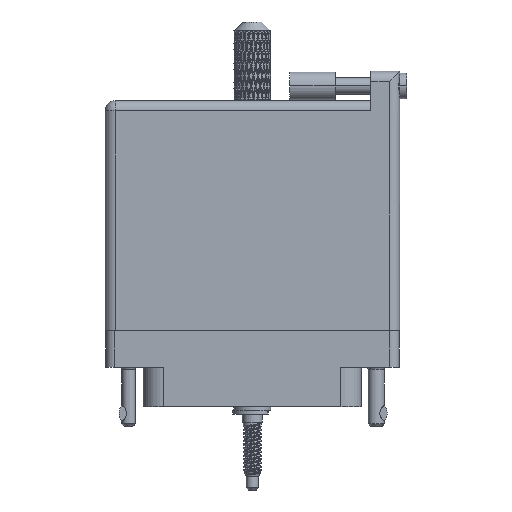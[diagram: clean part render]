
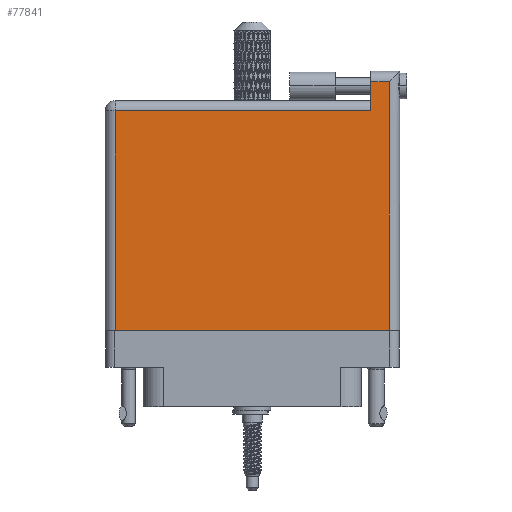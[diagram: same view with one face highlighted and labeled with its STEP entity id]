
A CAD part, front view. The second image highlights one B-rep face of the part: STEP entity #77841.
In plain terms, the highlighted face is planar.
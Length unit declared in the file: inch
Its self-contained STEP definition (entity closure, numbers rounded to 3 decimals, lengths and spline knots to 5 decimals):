
#797 = AXIS2_PLACEMENT_3D ( 'NONE', #28950, #56040, #91653 ) ;
#2466 = VERTEX_POINT ( 'NONE', #64165 ) ;
#3136 = ORIENTED_EDGE ( 'NONE', *, *, #99495, .T. ) ;
#6289 = LINE ( 'NONE', #6969, #58977 ) ;
#6969 = CARTESIAN_POINT ( 'NONE',  ( -1.004, 1.596, 0.4495 ) ) ;
#8138 = LINE ( 'NONE', #91094, #111970 ) ;
#11871 = PLANE ( 'NONE',  #797 ) ;
#13408 = VERTEX_POINT ( 'NONE', #24017 ) ;
#19342 = VERTEX_POINT ( 'NONE', #35663 ) ;
#21701 = EDGE_CURVE ( 'NONE', #56853, #80754, #68148, .T. ) ;
#23378 = CARTESIAN_POINT ( 'NONE',  ( -0.934, -0.1, 0.4495 ) ) ;
#24017 = CARTESIAN_POINT ( 'NONE',  ( 0.807, 1.596, 0.4495 ) ) ;
#25613 = ORIENTED_EDGE ( 'NONE', *, *, #74260, .T. ) ;
#26978 = ORIENTED_EDGE ( 'NONE', *, *, #79634, .T. ) ;
#27271 = ORIENTED_EDGE ( 'NONE', *, *, #21701, .T. ) ;
#28950 = CARTESIAN_POINT ( 'NONE',  ( -1.004, 1.466, 0.4495 ) ) ;
#33632 = LINE ( 'NONE', #95718, #86313 ) ;
#34148 = DIRECTION ( 'NONE',  ( 0., 1., 0. ) ) ;
#35663 = CARTESIAN_POINT ( 'NONE',  ( 0.807, 1.396, 0.4495 ) ) ;
#43052 = VERTEX_POINT ( 'NONE', #74578 ) ;
#43727 = CARTESIAN_POINT ( 'NONE',  ( -1.004, 1.396, 0.4495 ) ) ;
#43791 = ORIENTED_EDGE ( 'NONE', *, *, #59577, .T. ) ;
#44895 = DIRECTION ( 'NONE',  ( 0., -1., 0. ) ) ;
#51412 = EDGE_LOOP ( 'NONE', ( #43791, #25613, #26978, #58460, #3136, #27271 ) ) ;
#53450 = CARTESIAN_POINT ( 'NONE',  ( -0.934, -0.1, 0.4495 ) ) ;
#56040 = DIRECTION ( 'NONE',  ( 0., 0., -1. ) ) ;
#56853 = VERTEX_POINT ( 'NONE', #70923 ) ;
#58460 = ORIENTED_EDGE ( 'NONE', *, *, #112462, .T. ) ;
#58977 = VECTOR ( 'NONE', #87895, 39.37008 ) ;
#59248 = CARTESIAN_POINT ( 'NONE',  ( -1.004, -0.1, 0.4495 ) ) ;
#59577 = EDGE_CURVE ( 'NONE', #80754, #2466, #71367, .T. ) ;
#60408 = DIRECTION ( 'NONE',  ( -1., 0., 0. ) ) ;
#64165 = CARTESIAN_POINT ( 'NONE',  ( 0.934, -0.1, 0.4495 ) ) ;
#67650 = FACE_OUTER_BOUND ( 'NONE', #51412, .T. ) ;
#68148 = LINE ( 'NONE', #53450, #84728 ) ;
#70923 = CARTESIAN_POINT ( 'NONE',  ( -0.934, 1.396, 0.4495 ) ) ;
#71240 = VECTOR ( 'NONE', #111097, 39.37008 ) ;
#71367 = LINE ( 'NONE', #59248, #71240 ) ;
#72909 = VECTOR ( 'NONE', #60408, 39.37008 ) ;
#74260 = EDGE_CURVE ( 'NONE', #2466, #43052, #33632, .T. ) ;
#74578 = CARTESIAN_POINT ( 'NONE',  ( 0.934, 1.596, 0.4495 ) ) ;
#77841 = ADVANCED_FACE ( 'NONE', ( #67650 ), #11871, .F. ) ;
#79634 = EDGE_CURVE ( 'NONE', #43052, #13408, #6289, .T. ) ;
#80754 = VERTEX_POINT ( 'NONE', #23378 ) ;
#84728 = VECTOR ( 'NONE', #44895, 39.37008 ) ;
#86313 = VECTOR ( 'NONE', #34148, 39.37008 ) ;
#87895 = DIRECTION ( 'NONE',  ( -1., 0., 0. ) ) ;
#91094 = CARTESIAN_POINT ( 'NONE',  ( 0.807, 1.666, 0.4495 ) ) ;
#91653 = DIRECTION ( 'NONE',  ( -1., 0., 0. ) ) ;
#95718 = CARTESIAN_POINT ( 'NONE',  ( 0.934, 1.666, 0.4495 ) ) ;
#99495 = EDGE_CURVE ( 'NONE', #19342, #56853, #104671, .T. ) ;
#101159 = DIRECTION ( 'NONE',  ( 0., -1., 0. ) ) ;
#104671 = LINE ( 'NONE', #43727, #72909 ) ;
#111097 = DIRECTION ( 'NONE',  ( 1., 0., 0. ) ) ;
#111970 = VECTOR ( 'NONE', #101159, 39.37008 ) ;
#112462 = EDGE_CURVE ( 'NONE', #13408, #19342, #8138, .T. ) ;
